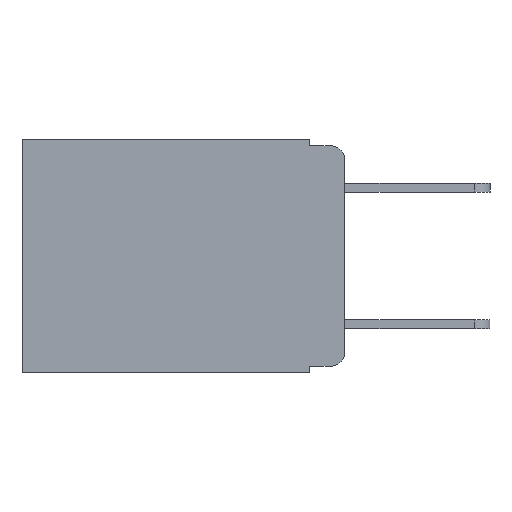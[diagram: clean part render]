
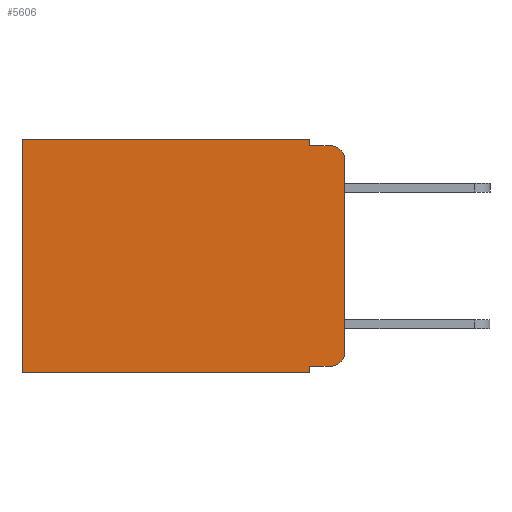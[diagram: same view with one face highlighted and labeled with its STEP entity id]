
A CAD part, left-side view. The second image highlights one B-rep face of the part: STEP entity #5606.
In plain terms, the highlighted planar face has unit normal (-1, 0, 0).
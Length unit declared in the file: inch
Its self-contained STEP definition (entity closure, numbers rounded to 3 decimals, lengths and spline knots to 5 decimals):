
#58 = CARTESIAN_POINT ( 'NONE',  ( 0.298, 0.051, 0. ) ) ;
#521 = EDGE_CURVE ( 'NONE', #3898, #6858, #7778, .T. ) ;
#583 = CARTESIAN_POINT ( 'NONE',  ( 0.298, 0.02, -0.313 ) ) ;
#820 = DIRECTION ( 'NONE',  ( 0., 0., -1. ) ) ;
#1058 = CARTESIAN_POINT ( 'NONE',  ( 0.298, 0.473, 0. ) ) ;
#1236 = CARTESIAN_POINT ( 'NONE',  ( 0.298, 0.02, -0.03 ) ) ;
#1335 = DIRECTION ( 'NONE',  ( 0., 0., -1. ) ) ;
#1372 = VERTEX_POINT ( 'NONE', #8997 ) ;
#1660 = LINE ( 'NONE', #5320, #8894 ) ;
#2026 = DIRECTION ( 'NONE',  ( 0., 0., -1. ) ) ;
#2186 = EDGE_CURVE ( 'NONE', #5922, #4669, #5250, .T. ) ;
#2189 = CARTESIAN_POINT ( 'NONE',  ( 0.298, 0.051, 0. ) ) ;
#2348 = DIRECTION ( 'NONE',  ( 0., 0., -1. ) ) ;
#2844 = VECTOR ( 'NONE', #820, 39.37008 ) ;
#2965 = CIRCLE ( 'NONE', #7894, 0.02 ) ;
#3155 = ORIENTED_EDGE ( 'NONE', *, *, #6625, .F. ) ;
#3174 = ORIENTED_EDGE ( 'NONE', *, *, #3890, .T. ) ;
#3203 = ORIENTED_EDGE ( 'NONE', *, *, #521, .T. ) ;
#3266 = CARTESIAN_POINT ( 'NONE',  ( 0.298, 0., -0.03 ) ) ;
#3273 = DIRECTION ( 'NONE',  ( 0., 0., -1. ) ) ;
#3285 = VECTOR ( 'NONE', #5100, 39.37008 ) ;
#3438 = DIRECTION ( 'NONE',  ( 0., 1., 0. ) ) ;
#3482 = ORIENTED_EDGE ( 'NONE', *, *, #7434, .F. ) ;
#3643 = EDGE_CURVE ( 'NONE', #9064, #8592, #7303, .T. ) ;
#3672 = CARTESIAN_POINT ( 'NONE',  ( 0.298, 0.02, -0.01 ) ) ;
#3692 = ORIENTED_EDGE ( 'NONE', *, *, #8727, .F. ) ;
#3766 = LINE ( 'NONE', #2189, #7593 ) ;
#3890 = EDGE_CURVE ( 'NONE', #1372, #3898, #1660, .T. ) ;
#3898 = VERTEX_POINT ( 'NONE', #4768 ) ;
#3914 = CARTESIAN_POINT ( 'NONE',  ( 0.298, 0.051, -0.01 ) ) ;
#3929 = CARTESIAN_POINT ( 'NONE',  ( 0.298, 0.051, -0.343 ) ) ;
#3965 = VECTOR ( 'NONE', #3438, 39.37008 ) ;
#3995 = AXIS2_PLACEMENT_3D ( 'NONE', #4594, #4560, #3273 ) ;
#4175 = CARTESIAN_POINT ( 'NONE',  ( 0.298, 0., -0.313 ) ) ;
#4325 = VERTEX_POINT ( 'NONE', #3929 ) ;
#4398 = VERTEX_POINT ( 'NONE', #4175 ) ;
#4510 = ORIENTED_EDGE ( 'NONE', *, *, #2186, .T. ) ;
#4560 = DIRECTION ( 'NONE',  ( 1., 0., 0. ) ) ;
#4594 = CARTESIAN_POINT ( 'NONE',  ( 0.298, 0., 0. ) ) ;
#4661 = ORIENTED_EDGE ( 'NONE', *, *, #7162, .T. ) ;
#4669 = VERTEX_POINT ( 'NONE', #9037 ) ;
#4731 = PLANE ( 'NONE',  #3995 ) ;
#4736 = DIRECTION ( 'NONE',  ( 0., 1., 0. ) ) ;
#4768 = CARTESIAN_POINT ( 'NONE',  ( 0.298, 0.473, 0. ) ) ;
#4814 = CARTESIAN_POINT ( 'NONE',  ( 0.298, 0.051, -0.01 ) ) ;
#4984 = DIRECTION ( 'NONE',  ( 0., 0., -1. ) ) ;
#5100 = DIRECTION ( 'NONE',  ( 0., -1., 0. ) ) ;
#5111 = CARTESIAN_POINT ( 'NONE',  ( 0.298, 0.051, -0.333 ) ) ;
#5250 = LINE ( 'NONE', #5111, #3285 ) ;
#5320 = CARTESIAN_POINT ( 'NONE',  ( 0.298, 0., 0. ) ) ;
#5606 = ADVANCED_FACE ( 'NONE', ( #5653 ), #4731, .F. ) ;
#5653 = FACE_OUTER_BOUND ( 'NONE', #7301, .T. ) ;
#5796 = DIRECTION ( 'NONE',  ( -1., 0., 0. ) ) ;
#5922 = VERTEX_POINT ( 'NONE', #7948 ) ;
#6024 = VECTOR ( 'NONE', #4984, 39.37008 ) ;
#6060 = ORIENTED_EDGE ( 'NONE', *, *, #6755, .F. ) ;
#6122 = VERTEX_POINT ( 'NONE', #3266 ) ;
#6162 = LINE ( 'NONE', #7331, #6780 ) ;
#6398 = DIRECTION ( 'NONE',  ( -1., 0., 0. ) ) ;
#6625 = EDGE_CURVE ( 'NONE', #1372, #9064, #3766, .T. ) ;
#6755 = EDGE_CURVE ( 'NONE', #6122, #4398, #6162, .T. ) ;
#6778 = ORIENTED_EDGE ( 'NONE', *, *, #8535, .T. ) ;
#6780 = VECTOR ( 'NONE', #2348, 39.37008 ) ;
#6811 = ORIENTED_EDGE ( 'NONE', *, *, #3643, .F. ) ;
#6858 = VERTEX_POINT ( 'NONE', #8115 ) ;
#6918 = CARTESIAN_POINT ( 'NONE',  ( 0.298, 0., -0.343 ) ) ;
#7162 = EDGE_CURVE ( 'NONE', #4669, #4398, #8111, .T. ) ;
#7175 = LINE ( 'NONE', #6918, #3965 ) ;
#7195 = DIRECTION ( 'NONE',  ( 0., 0., -1. ) ) ;
#7301 = EDGE_LOOP ( 'NONE', ( #6060, #6778, #6811, #3155, #3174, #3203, #3482, #3692, #4510, #4661 ) ) ;
#7303 = LINE ( 'NONE', #4814, #8795 ) ;
#7331 = CARTESIAN_POINT ( 'NONE',  ( 0.298, 0., 0. ) ) ;
#7367 = DIRECTION ( 'NONE',  ( 0., -1., 0. ) ) ;
#7434 = EDGE_CURVE ( 'NONE', #4325, #6858, #7175, .T. ) ;
#7593 = VECTOR ( 'NONE', #7195, 39.37008 ) ;
#7778 = LINE ( 'NONE', #1058, #6024 ) ;
#7894 = AXIS2_PLACEMENT_3D ( 'NONE', #1236, #6398, #2026 ) ;
#7948 = CARTESIAN_POINT ( 'NONE',  ( 0.298, 0.051, -0.333 ) ) ;
#8108 = AXIS2_PLACEMENT_3D ( 'NONE', #583, #5796, #1335 ) ;
#8111 = CIRCLE ( 'NONE', #8108, 0.02 ) ;
#8115 = CARTESIAN_POINT ( 'NONE',  ( 0.298, 0.473, -0.343 ) ) ;
#8368 = LINE ( 'NONE', #58, #2844 ) ;
#8535 = EDGE_CURVE ( 'NONE', #6122, #8592, #2965, .T. ) ;
#8592 = VERTEX_POINT ( 'NONE', #3672 ) ;
#8727 = EDGE_CURVE ( 'NONE', #5922, #4325, #8368, .T. ) ;
#8795 = VECTOR ( 'NONE', #7367, 39.37008 ) ;
#8894 = VECTOR ( 'NONE', #4736, 39.37008 ) ;
#8997 = CARTESIAN_POINT ( 'NONE',  ( 0.298, 0.051, 0. ) ) ;
#9037 = CARTESIAN_POINT ( 'NONE',  ( 0.298, 0.02, -0.333 ) ) ;
#9064 = VERTEX_POINT ( 'NONE', #3914 ) ;
